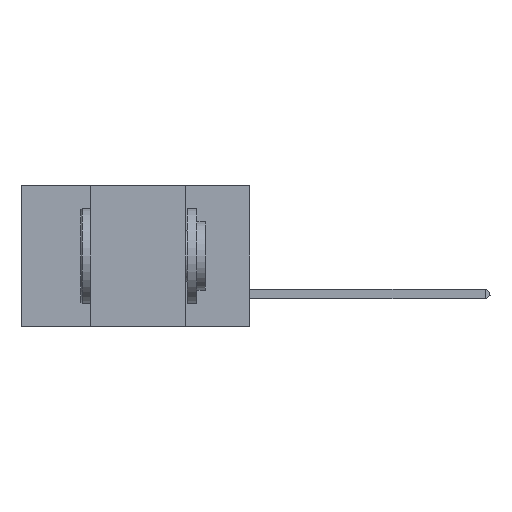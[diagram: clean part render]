
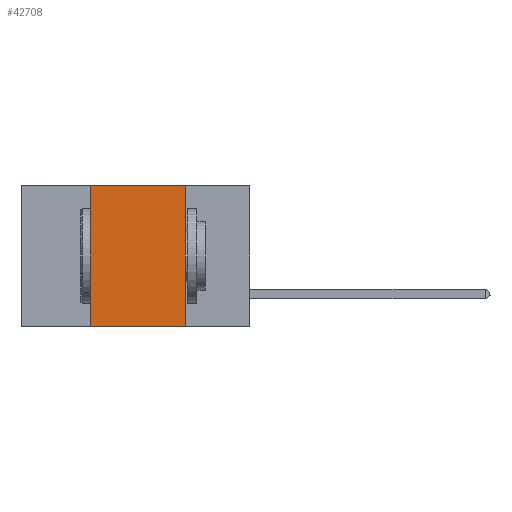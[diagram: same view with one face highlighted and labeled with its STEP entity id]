
A CAD part, left-side view. The second image highlights one B-rep face of the part: STEP entity #42708.
In plain terms, the highlighted planar face has unit normal (-1, 0, 0).
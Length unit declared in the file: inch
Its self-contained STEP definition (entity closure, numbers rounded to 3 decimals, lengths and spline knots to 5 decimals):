
#303 = EDGE_CURVE ( 'NONE', #26851, #46717, #5208, .T. ) ;
#956 = VECTOR ( 'NONE', #14091, 39.37008 ) ;
#2307 = VECTOR ( 'NONE', #33363, 39.37008 ) ;
#2347 = EDGE_CURVE ( 'NONE', #34316, #46717, #22453, .T. ) ;
#2613 = LINE ( 'NONE', #29332, #29259 ) ;
#5093 = DIRECTION ( 'NONE',  ( 1., 0., 0. ) ) ;
#5208 = LINE ( 'NONE', #33691, #2307 ) ;
#6932 = ORIENTED_EDGE ( 'NONE', *, *, #13649, .F. ) ;
#8643 = ORIENTED_EDGE ( 'NONE', *, *, #303, .T. ) ;
#8856 = EDGE_CURVE ( 'NONE', #26851, #18948, #2613, .T. ) ;
#10588 = VECTOR ( 'NONE', #40565, 39.37008 ) ;
#10673 = CARTESIAN_POINT ( 'NONE',  ( 0., 0.42, -0.37 ) ) ;
#12642 = EDGE_LOOP ( 'NONE', ( #30503, #6932, #32435, #8643 ) ) ;
#13649 = EDGE_CURVE ( 'NONE', #18948, #34316, #18711, .T. ) ;
#14091 = DIRECTION ( 'NONE',  ( 0., -1., 0. ) ) ;
#16704 = CARTESIAN_POINT ( 'NONE',  ( 0., 0.6, 0. ) ) ;
#18711 = LINE ( 'NONE', #24068, #956 ) ;
#18948 = VERTEX_POINT ( 'NONE', #40700 ) ;
#22453 = LINE ( 'NONE', #44236, #10588 ) ;
#24068 = CARTESIAN_POINT ( 'NONE',  ( 0., 0.6, 0. ) ) ;
#24850 = CARTESIAN_POINT ( 'NONE',  ( 0., 0.17, -0.37 ) ) ;
#26851 = VERTEX_POINT ( 'NONE', #10673 ) ;
#29259 = VECTOR ( 'NONE', #48734, 39.37008 ) ;
#29332 = CARTESIAN_POINT ( 'NONE',  ( 0., 0.42, 0. ) ) ;
#30503 = ORIENTED_EDGE ( 'NONE', *, *, #2347, .F. ) ;
#32435 = ORIENTED_EDGE ( 'NONE', *, *, #8856, .F. ) ;
#33363 = DIRECTION ( 'NONE',  ( 0., -1., 0. ) ) ;
#33460 = CARTESIAN_POINT ( 'NONE',  ( 0., 0.17, 0. ) ) ;
#33691 = CARTESIAN_POINT ( 'NONE',  ( 0., 0.6, -0.37 ) ) ;
#33774 = AXIS2_PLACEMENT_3D ( 'NONE', #16704, #5093, #35381 ) ;
#34316 = VERTEX_POINT ( 'NONE', #33460 ) ;
#35381 = DIRECTION ( 'NONE',  ( 0., 0., -1. ) ) ;
#40565 = DIRECTION ( 'NONE',  ( 0., 0., -1. ) ) ;
#40700 = CARTESIAN_POINT ( 'NONE',  ( 0., 0.42, 0. ) ) ;
#42708 = ADVANCED_FACE ( 'NONE', ( #48910 ), #43025, .F. ) ;
#43025 = PLANE ( 'NONE',  #33774 ) ;
#44236 = CARTESIAN_POINT ( 'NONE',  ( 0., 0.17, 0. ) ) ;
#46717 = VERTEX_POINT ( 'NONE', #24850 ) ;
#48734 = DIRECTION ( 'NONE',  ( 0., 0., 1. ) ) ;
#48910 = FACE_OUTER_BOUND ( 'NONE', #12642, .T. ) ;
